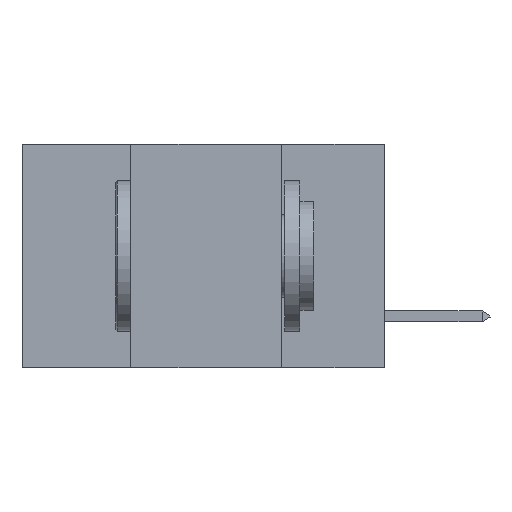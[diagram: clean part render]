
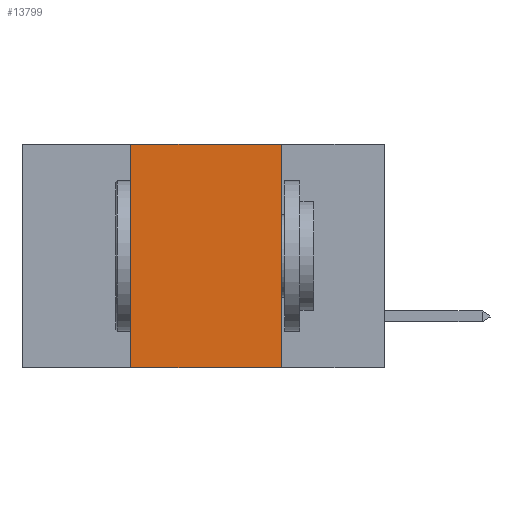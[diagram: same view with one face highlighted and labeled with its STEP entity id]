
A CAD part, left-side view. The second image highlights one B-rep face of the part: STEP entity #13799.
In plain terms, the highlighted planar face has unit normal (-1, 0, 0).
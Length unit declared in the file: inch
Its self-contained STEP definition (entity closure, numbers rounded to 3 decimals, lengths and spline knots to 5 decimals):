
#1438 = CARTESIAN_POINT ( 'NONE',  ( 0., 0.17, 0. ) ) ;
#1904 = EDGE_LOOP ( 'NONE', ( #8280, #9468, #6758, #16127 ) ) ;
#3039 = CARTESIAN_POINT ( 'NONE',  ( 0., 0.6, 0. ) ) ;
#3364 = DIRECTION ( 'NONE',  ( 0., 0., 1. ) ) ;
#4429 = CARTESIAN_POINT ( 'NONE',  ( 0., 0.6, 0. ) ) ;
#5024 = EDGE_CURVE ( 'NONE', #11059, #14745, #16523, .T. ) ;
#5739 = CARTESIAN_POINT ( 'NONE',  ( 0., 0.17, 0. ) ) ;
#6226 = CARTESIAN_POINT ( 'NONE',  ( 0., 0.42, 0. ) ) ;
#6488 = DIRECTION ( 'NONE',  ( 0., -1., 0. ) ) ;
#6758 = ORIENTED_EDGE ( 'NONE', *, *, #16728, .F. ) ;
#6985 = EDGE_CURVE ( 'NONE', #9880, #14745, #9367, .T. ) ;
#7141 = VECTOR ( 'NONE', #10906, 39.37008 ) ;
#7288 = VECTOR ( 'NONE', #3364, 39.37008 ) ;
#7528 = LINE ( 'NONE', #4429, #12859 ) ;
#7663 = CARTESIAN_POINT ( 'NONE',  ( 0., 0.42, 0. ) ) ;
#8280 = ORIENTED_EDGE ( 'NONE', *, *, #5024, .F. ) ;
#9367 = LINE ( 'NONE', #10574, #10819 ) ;
#9468 = ORIENTED_EDGE ( 'NONE', *, *, #16320, .F. ) ;
#9744 = AXIS2_PLACEMENT_3D ( 'NONE', #3039, #14017, #16697 ) ;
#9880 = VERTEX_POINT ( 'NONE', #11228 ) ;
#9904 = DIRECTION ( 'NONE',  ( 0., -1., 0. ) ) ;
#10574 = CARTESIAN_POINT ( 'NONE',  ( 0., 0.6, -0.37 ) ) ;
#10794 = VERTEX_POINT ( 'NONE', #6226 ) ;
#10819 = VECTOR ( 'NONE', #6488, 39.37008 ) ;
#10906 = DIRECTION ( 'NONE',  ( 0., 0., -1. ) ) ;
#11059 = VERTEX_POINT ( 'NONE', #5739 ) ;
#11228 = CARTESIAN_POINT ( 'NONE',  ( 0., 0.42, -0.37 ) ) ;
#11591 = CARTESIAN_POINT ( 'NONE',  ( 0., 0.17, -0.37 ) ) ;
#12324 = FACE_OUTER_BOUND ( 'NONE', #1904, .T. ) ;
#12859 = VECTOR ( 'NONE', #9904, 39.37008 ) ;
#13799 = ADVANCED_FACE ( 'NONE', ( #12324 ), #16580, .F. ) ;
#14017 = DIRECTION ( 'NONE',  ( 1., 0., 0. ) ) ;
#14560 = LINE ( 'NONE', #7663, #7288 ) ;
#14745 = VERTEX_POINT ( 'NONE', #11591 ) ;
#16127 = ORIENTED_EDGE ( 'NONE', *, *, #6985, .T. ) ;
#16320 = EDGE_CURVE ( 'NONE', #10794, #11059, #7528, .T. ) ;
#16523 = LINE ( 'NONE', #1438, #7141 ) ;
#16580 = PLANE ( 'NONE',  #9744 ) ;
#16697 = DIRECTION ( 'NONE',  ( 0., 0., -1. ) ) ;
#16728 = EDGE_CURVE ( 'NONE', #9880, #10794, #14560, .T. ) ;
